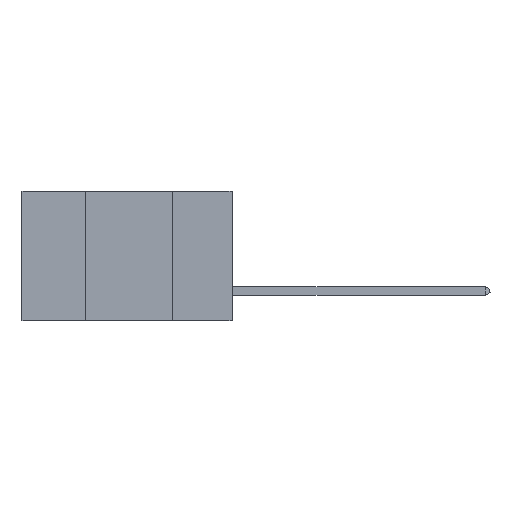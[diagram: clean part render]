
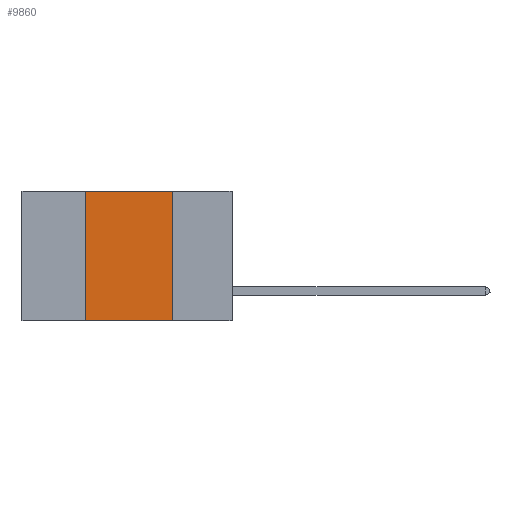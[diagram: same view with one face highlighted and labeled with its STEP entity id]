
A CAD part, left-side view. The second image highlights one B-rep face of the part: STEP entity #9860.
In plain terms, the highlighted planar face has unit normal (-1, 0, 0).
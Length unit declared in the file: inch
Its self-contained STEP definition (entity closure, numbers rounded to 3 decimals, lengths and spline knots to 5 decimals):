
#153 = FACE_OUTER_BOUND ( 'NONE', #13865, .T. ) ;
#1311 = ORIENTED_EDGE ( 'NONE', *, *, #3110, .F. ) ;
#1858 = LINE ( 'NONE', #12789, #8646 ) ;
#2419 = CARTESIAN_POINT ( 'NONE',  ( 0., 0.17, -0.37 ) ) ;
#2551 = CARTESIAN_POINT ( 'NONE',  ( 0., 0.6, 0. ) ) ;
#2577 = DIRECTION ( 'NONE',  ( 0., 0., -1. ) ) ;
#2620 = EDGE_CURVE ( 'NONE', #7552, #8173, #5784, .T. ) ;
#3110 = EDGE_CURVE ( 'NONE', #9347, #7552, #1858, .T. ) ;
#4324 = LINE ( 'NONE', #11178, #8729 ) ;
#4388 = AXIS2_PLACEMENT_3D ( 'NONE', #2551, #7459, #4762 ) ;
#4762 = DIRECTION ( 'NONE',  ( 0., 0., -1. ) ) ;
#4919 = PLANE ( 'NONE',  #4388 ) ;
#5105 = ORIENTED_EDGE ( 'NONE', *, *, #11218, .F. ) ;
#5784 = LINE ( 'NONE', #12722, #13639 ) ;
#6815 = DIRECTION ( 'NONE',  ( 0., 0., 1. ) ) ;
#7459 = DIRECTION ( 'NONE',  ( 1., 0., 0. ) ) ;
#7552 = VERTEX_POINT ( 'NONE', #9068 ) ;
#7622 = VERTEX_POINT ( 'NONE', #2419 ) ;
#8173 = VERTEX_POINT ( 'NONE', #13525 ) ;
#8354 = ORIENTED_EDGE ( 'NONE', *, *, #14565, .T. ) ;
#8555 = ORIENTED_EDGE ( 'NONE', *, *, #2620, .F. ) ;
#8646 = VECTOR ( 'NONE', #6815, 39.37008 ) ;
#8729 = VECTOR ( 'NONE', #11258, 39.37008 ) ;
#9068 = CARTESIAN_POINT ( 'NONE',  ( 0., 0.42, 0. ) ) ;
#9347 = VERTEX_POINT ( 'NONE', #14483 ) ;
#9860 = ADVANCED_FACE ( 'NONE', ( #153 ), #4919, .F. ) ;
#9899 = LINE ( 'NONE', #12512, #14961 ) ;
#11178 = CARTESIAN_POINT ( 'NONE',  ( 0., 0.6, -0.37 ) ) ;
#11218 = EDGE_CURVE ( 'NONE', #8173, #7622, #9899, .T. ) ;
#11258 = DIRECTION ( 'NONE',  ( 0., -1., 0. ) ) ;
#12512 = CARTESIAN_POINT ( 'NONE',  ( 0., 0.17, 0. ) ) ;
#12722 = CARTESIAN_POINT ( 'NONE',  ( 0., 0.6, 0. ) ) ;
#12789 = CARTESIAN_POINT ( 'NONE',  ( 0., 0.42, 0. ) ) ;
#13525 = CARTESIAN_POINT ( 'NONE',  ( 0., 0.17, 0. ) ) ;
#13639 = VECTOR ( 'NONE', #15066, 39.37008 ) ;
#13865 = EDGE_LOOP ( 'NONE', ( #5105, #8555, #1311, #8354 ) ) ;
#14483 = CARTESIAN_POINT ( 'NONE',  ( 0., 0.42, -0.37 ) ) ;
#14565 = EDGE_CURVE ( 'NONE', #9347, #7622, #4324, .T. ) ;
#14961 = VECTOR ( 'NONE', #2577, 39.37008 ) ;
#15066 = DIRECTION ( 'NONE',  ( 0., -1., 0. ) ) ;
